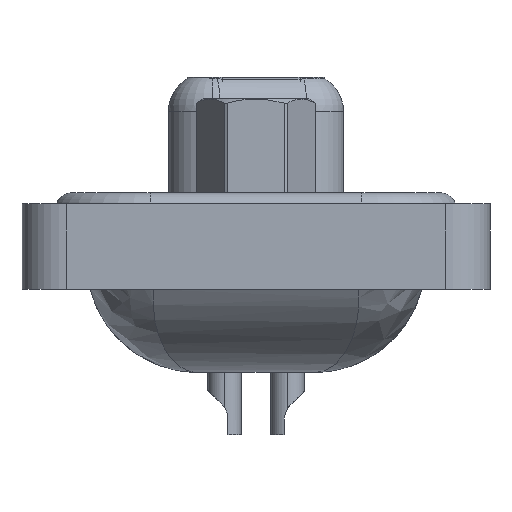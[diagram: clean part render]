
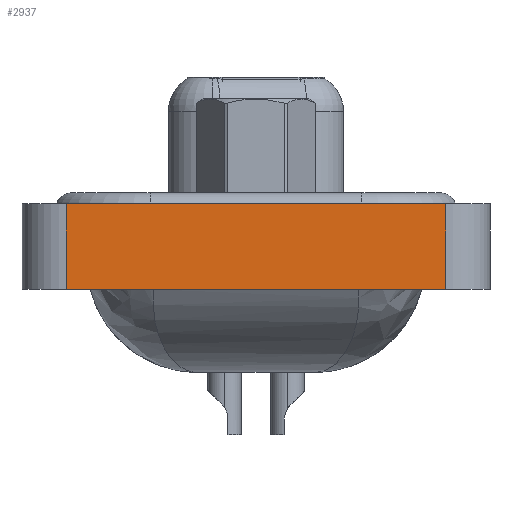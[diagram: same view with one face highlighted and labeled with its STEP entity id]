
A CAD part, left-side view. The second image highlights one B-rep face of the part: STEP entity #2937.
In plain terms, the highlighted planar face has unit normal (-1, 0, 0).
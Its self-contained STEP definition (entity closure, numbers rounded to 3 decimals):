
#6 = CARTESIAN_POINT ( 'NONE',  ( -7.25, -8.55, 0.5 ) ) ;
#111 = LINE ( 'NONE', #6800, #7265 ) ;
#696 = VECTOR ( 'NONE', #16813, 1000. ) ;
#733 = AXIS2_PLACEMENT_3D ( 'NONE', #9558, #14916, #15026 ) ;
#761 = EDGE_CURVE ( 'NONE', #5954, #16623, #13410, .T. ) ;
#2521 = CARTESIAN_POINT ( 'NONE',  ( -7.25, -8.55, -3.35 ) ) ;
#2937 = ADVANCED_FACE ( 'NONE', ( #19575 ), #11190, .T. ) ;
#2993 = VERTEX_POINT ( 'NONE', #6 ) ;
#3091 = ORIENTED_EDGE ( 'NONE', *, *, #20511, .F. ) ;
#4284 = ORIENTED_EDGE ( 'NONE', *, *, #14953, .F. ) ;
#5954 = VERTEX_POINT ( 'NONE', #6226 ) ;
#6182 = VECTOR ( 'NONE', #13089, 1000. ) ;
#6226 = CARTESIAN_POINT ( 'NONE',  ( -7.25, 8.55, -3.35 ) ) ;
#6693 = CARTESIAN_POINT ( 'NONE',  ( -7.25, -8.55, -3.35 ) ) ;
#6800 = CARTESIAN_POINT ( 'NONE',  ( -7.25, -8.55, 0.5 ) ) ;
#7265 = VECTOR ( 'NONE', #15018, 1000. ) ;
#7780 = VERTEX_POINT ( 'NONE', #8812 ) ;
#8812 = CARTESIAN_POINT ( 'NONE',  ( -7.25, 8.55, 0.5 ) ) ;
#9207 = DIRECTION ( 'NONE',  ( 0., 0., 1. ) ) ;
#9332 = EDGE_LOOP ( 'NONE', ( #11900, #3091, #4284, #19774 ) ) ;
#9558 = CARTESIAN_POINT ( 'NONE',  ( -7.25, -8.55, -3.35 ) ) ;
#11184 = EDGE_CURVE ( 'NONE', #16623, #2993, #17339, .T. ) ;
#11190 = PLANE ( 'NONE',  #733 ) ;
#11900 = ORIENTED_EDGE ( 'NONE', *, *, #11184, .T. ) ;
#11955 = LINE ( 'NONE', #15484, #696 ) ;
#13089 = DIRECTION ( 'NONE',  ( 0., -1., 0. ) ) ;
#13410 = LINE ( 'NONE', #19912, #6182 ) ;
#14916 = DIRECTION ( 'NONE',  ( -1., 0., 0. ) ) ;
#14953 = EDGE_CURVE ( 'NONE', #5954, #7780, #11955, .T. ) ;
#15018 = DIRECTION ( 'NONE',  ( 0., -1., 0. ) ) ;
#15026 = DIRECTION ( 'NONE',  ( 0., 0., 1. ) ) ;
#15484 = CARTESIAN_POINT ( 'NONE',  ( -7.25, 8.55, -3.35 ) ) ;
#16623 = VERTEX_POINT ( 'NONE', #6693 ) ;
#16813 = DIRECTION ( 'NONE',  ( 0., 0., 1. ) ) ;
#17339 = LINE ( 'NONE', #2521, #21585 ) ;
#19575 = FACE_OUTER_BOUND ( 'NONE', #9332, .T. ) ;
#19774 = ORIENTED_EDGE ( 'NONE', *, *, #761, .T. ) ;
#19912 = CARTESIAN_POINT ( 'NONE',  ( -7.25, -8.55, -3.35 ) ) ;
#20511 = EDGE_CURVE ( 'NONE', #7780, #2993, #111, .T. ) ;
#21585 = VECTOR ( 'NONE', #9207, 1000. ) ;
